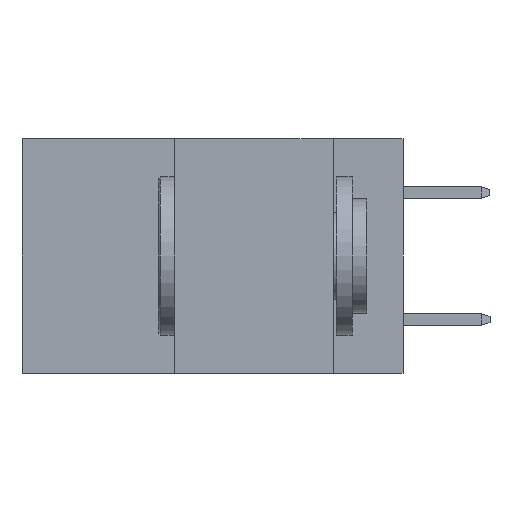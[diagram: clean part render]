
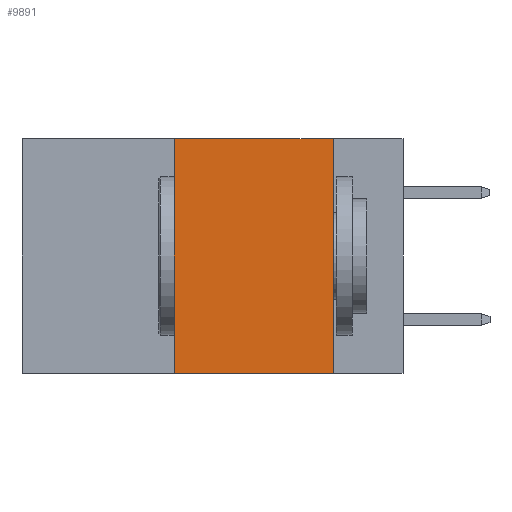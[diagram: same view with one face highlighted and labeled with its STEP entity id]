
A CAD part, left-side view. The second image highlights one B-rep face of the part: STEP entity #9891.
In plain terms, the highlighted planar face has unit normal (-1, 0, 0).
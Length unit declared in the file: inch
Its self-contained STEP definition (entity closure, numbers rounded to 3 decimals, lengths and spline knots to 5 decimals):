
#701 = DIRECTION ( 'NONE',  ( 0., -1., 0. ) ) ;
#813 = FACE_OUTER_BOUND ( 'NONE', #7411, .T. ) ;
#1642 = DIRECTION ( 'NONE',  ( 1., 0., 0. ) ) ;
#1675 = CARTESIAN_POINT ( 'NONE',  ( 0., 0.36, 0. ) ) ;
#2006 = EDGE_CURVE ( 'NONE', #2911, #13189, #3882, .T. ) ;
#2270 = ORIENTED_EDGE ( 'NONE', *, *, #7924, .T. ) ;
#2911 = VERTEX_POINT ( 'NONE', #1675 ) ;
#3882 = LINE ( 'NONE', #5167, #3945 ) ;
#3945 = VECTOR ( 'NONE', #701, 39.37008 ) ;
#4030 = LINE ( 'NONE', #7133, #9003 ) ;
#4431 = ORIENTED_EDGE ( 'NONE', *, *, #2006, .F. ) ;
#5054 = DIRECTION ( 'NONE',  ( 0., 0., 1. ) ) ;
#5156 = ORIENTED_EDGE ( 'NONE', *, *, #9289, .F. ) ;
#5167 = CARTESIAN_POINT ( 'NONE',  ( 0., 0.6, 0. ) ) ;
#5696 = VECTOR ( 'NONE', #6185, 39.37008 ) ;
#6185 = DIRECTION ( 'NONE',  ( 0., 0., -1. ) ) ;
#7133 = CARTESIAN_POINT ( 'NONE',  ( 0., 0.36, 0. ) ) ;
#7411 = EDGE_LOOP ( 'NONE', ( #5156, #4431, #7414, #2270 ) ) ;
#7414 = ORIENTED_EDGE ( 'NONE', *, *, #8435, .F. ) ;
#7924 = EDGE_CURVE ( 'NONE', #13088, #10505, #8964, .T. ) ;
#7956 = CARTESIAN_POINT ( 'NONE',  ( 0., 0.6, 0. ) ) ;
#8435 = EDGE_CURVE ( 'NONE', #13088, #2911, #4030, .T. ) ;
#8964 = LINE ( 'NONE', #10267, #13390 ) ;
#9003 = VECTOR ( 'NONE', #5054, 39.37008 ) ;
#9129 = CARTESIAN_POINT ( 'NONE',  ( 0., 0.11, 0. ) ) ;
#9269 = PLANE ( 'NONE',  #11877 ) ;
#9289 = EDGE_CURVE ( 'NONE', #13189, #10505, #9578, .T. ) ;
#9578 = LINE ( 'NONE', #12451, #5696 ) ;
#9891 = ADVANCED_FACE ( 'NONE', ( #813 ), #9269, .F. ) ;
#10267 = CARTESIAN_POINT ( 'NONE',  ( 0., 0.6, -0.37 ) ) ;
#10505 = VERTEX_POINT ( 'NONE', #13255 ) ;
#11877 = AXIS2_PLACEMENT_3D ( 'NONE', #7956, #1642, #13400 ) ;
#12119 = DIRECTION ( 'NONE',  ( 0., -1., 0. ) ) ;
#12451 = CARTESIAN_POINT ( 'NONE',  ( 0., 0.11, 0. ) ) ;
#13049 = CARTESIAN_POINT ( 'NONE',  ( 0., 0.36, -0.37 ) ) ;
#13088 = VERTEX_POINT ( 'NONE', #13049 ) ;
#13189 = VERTEX_POINT ( 'NONE', #9129 ) ;
#13255 = CARTESIAN_POINT ( 'NONE',  ( 0., 0.11, -0.37 ) ) ;
#13390 = VECTOR ( 'NONE', #12119, 39.37008 ) ;
#13400 = DIRECTION ( 'NONE',  ( 0., 0., -1. ) ) ;
